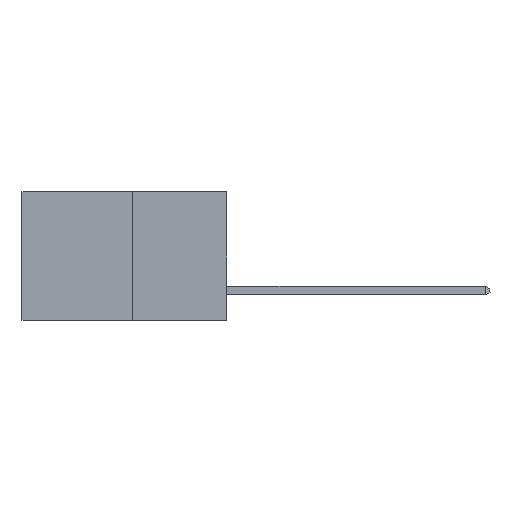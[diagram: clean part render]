
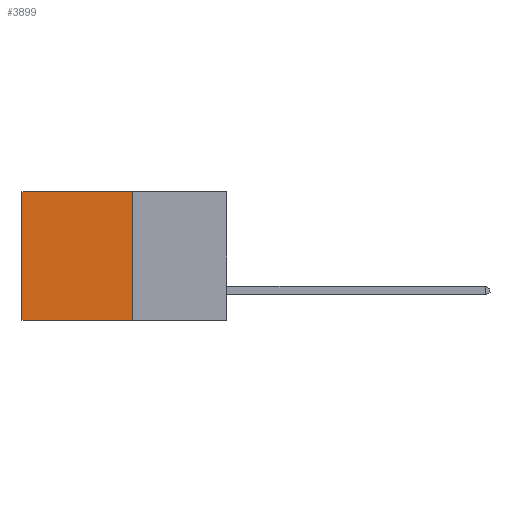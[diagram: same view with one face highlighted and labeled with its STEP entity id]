
A CAD part, left-side view. The second image highlights one B-rep face of the part: STEP entity #3899.
In plain terms, the highlighted planar face has unit normal (-1, 0, 0).
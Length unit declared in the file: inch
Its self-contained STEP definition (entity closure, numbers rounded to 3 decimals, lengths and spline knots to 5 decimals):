
#157 = DIRECTION ( 'NONE',  ( 1., 0., 0. ) ) ;
#754 = VERTEX_POINT ( 'NONE', #7315 ) ;
#846 = CARTESIAN_POINT ( 'NONE',  ( 0.277, 0.27, 0. ) ) ;
#1421 = EDGE_CURVE ( 'NONE', #5654, #5290, #7895, .T. ) ;
#1445 = VECTOR ( 'NONE', #7406, 39.37008 ) ;
#1850 = CARTESIAN_POINT ( 'NONE',  ( 0.277, 0.59, 0. ) ) ;
#1932 = ORIENTED_EDGE ( 'NONE', *, *, #9929, .T. ) ;
#2395 = EDGE_LOOP ( 'NONE', ( #1932, #7100, #7952, #4252 ) ) ;
#2550 = DIRECTION ( 'NONE',  ( 0., 0., -1. ) ) ;
#2594 = CARTESIAN_POINT ( 'NONE',  ( 0.277, 0.27, -0.37 ) ) ;
#2760 = CARTESIAN_POINT ( 'NONE',  ( 0.277, 0.27, -0.37 ) ) ;
#3170 = VERTEX_POINT ( 'NONE', #7762 ) ;
#3766 = VECTOR ( 'NONE', #4646, 39.37008 ) ;
#3899 = ADVANCED_FACE ( 'NONE', ( #5663 ), #4823, .F. ) ;
#4131 = EDGE_CURVE ( 'NONE', #754, #3170, #5328, .T. ) ;
#4252 = ORIENTED_EDGE ( 'NONE', *, *, #1421, .T. ) ;
#4646 = DIRECTION ( 'NONE',  ( 0., 1., 0. ) ) ;
#4823 = PLANE ( 'NONE',  #7814 ) ;
#4845 = CARTESIAN_POINT ( 'NONE',  ( 0.277, 0.59, -0.37 ) ) ;
#4902 = VECTOR ( 'NONE', #2550, 39.37008 ) ;
#5290 = VERTEX_POINT ( 'NONE', #1850 ) ;
#5328 = LINE ( 'NONE', #2760, #1445 ) ;
#5586 = CARTESIAN_POINT ( 'NONE',  ( 0.277, 0.27, -0.37 ) ) ;
#5616 = DIRECTION ( 'NONE',  ( 0., 0., -1. ) ) ;
#5654 = VERTEX_POINT ( 'NONE', #846 ) ;
#5663 = FACE_OUTER_BOUND ( 'NONE', #2395, .T. ) ;
#6264 = CARTESIAN_POINT ( 'NONE',  ( 0.277, 0.27, 0. ) ) ;
#6973 = LINE ( 'NONE', #4845, #4902 ) ;
#7100 = ORIENTED_EDGE ( 'NONE', *, *, #4131, .F. ) ;
#7151 = EDGE_CURVE ( 'NONE', #5654, #754, #8041, .T. ) ;
#7247 = DIRECTION ( 'NONE',  ( 0., 0., -1. ) ) ;
#7315 = CARTESIAN_POINT ( 'NONE',  ( 0.277, 0.27, -0.37 ) ) ;
#7406 = DIRECTION ( 'NONE',  ( 0., 1., 0. ) ) ;
#7762 = CARTESIAN_POINT ( 'NONE',  ( 0.277, 0.59, -0.37 ) ) ;
#7814 = AXIS2_PLACEMENT_3D ( 'NONE', #5586, #157, #5616 ) ;
#7895 = LINE ( 'NONE', #6264, #3766 ) ;
#7952 = ORIENTED_EDGE ( 'NONE', *, *, #7151, .F. ) ;
#8041 = LINE ( 'NONE', #2594, #8282 ) ;
#8282 = VECTOR ( 'NONE', #7247, 39.37008 ) ;
#9929 = EDGE_CURVE ( 'NONE', #5290, #3170, #6973, .T. ) ;
